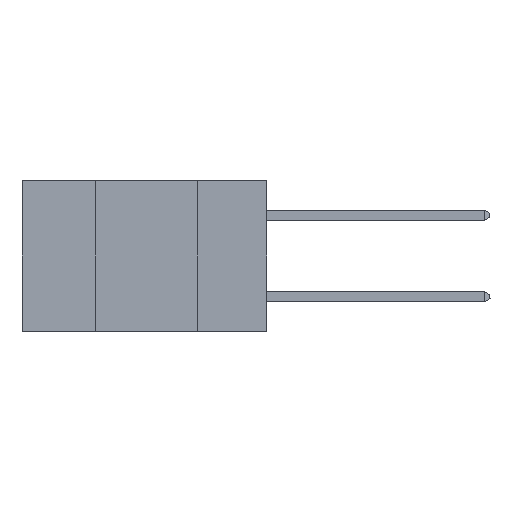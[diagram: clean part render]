
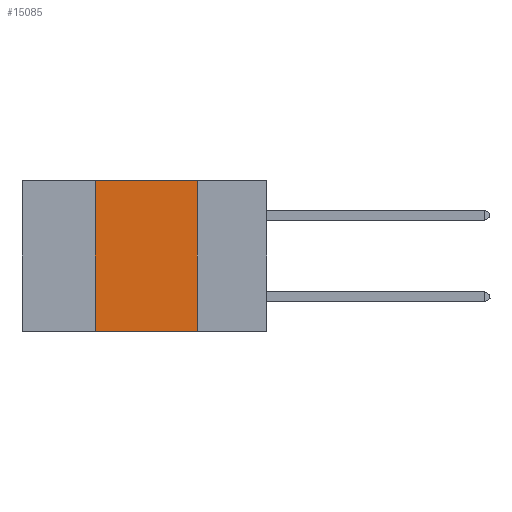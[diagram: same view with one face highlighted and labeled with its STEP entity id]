
A CAD part, left-side view. The second image highlights one B-rep face of the part: STEP entity #15085.
In plain terms, the highlighted planar face has unit normal (-1, 0, 0).
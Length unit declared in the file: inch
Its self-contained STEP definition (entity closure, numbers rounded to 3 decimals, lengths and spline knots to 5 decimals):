
#708 = CARTESIAN_POINT ( 'NONE',  ( 0., 0.6, -0.37 ) ) ;
#858 = CARTESIAN_POINT ( 'NONE',  ( 0., 0.42, 0. ) ) ;
#1692 = VECTOR ( 'NONE', #8683, 39.37008 ) ;
#1806 = ORIENTED_EDGE ( 'NONE', *, *, #21618, .F. ) ;
#2243 = PLANE ( 'NONE',  #3837 ) ;
#3837 = AXIS2_PLACEMENT_3D ( 'NONE', #10097, #6200, #8025 ) ;
#5369 = CARTESIAN_POINT ( 'NONE',  ( 0., 0.42, 0. ) ) ;
#6200 = DIRECTION ( 'NONE',  ( 1., 0., 0. ) ) ;
#6962 = VECTOR ( 'NONE', #6995, 39.37008 ) ;
#6995 = DIRECTION ( 'NONE',  ( 0., -1., 0. ) ) ;
#7097 = DIRECTION ( 'NONE',  ( 0., 0., 1. ) ) ;
#8025 = DIRECTION ( 'NONE',  ( 0., 0., -1. ) ) ;
#8031 = VECTOR ( 'NONE', #7097, 39.37008 ) ;
#8683 = DIRECTION ( 'NONE',  ( 0., -1., 0. ) ) ;
#8914 = CARTESIAN_POINT ( 'NONE',  ( 0., 0.42, -0.37 ) ) ;
#9021 = VERTEX_POINT ( 'NONE', #8914 ) ;
#9606 = EDGE_LOOP ( 'NONE', ( #1806, #12140, #15367, #12699 ) ) ;
#10015 = VERTEX_POINT ( 'NONE', #5369 ) ;
#10097 = CARTESIAN_POINT ( 'NONE',  ( 0., 0.6, 0. ) ) ;
#11702 = DIRECTION ( 'NONE',  ( 0., 0., -1. ) ) ;
#12140 = ORIENTED_EDGE ( 'NONE', *, *, #24425, .F. ) ;
#12699 = ORIENTED_EDGE ( 'NONE', *, *, #23178, .T. ) ;
#13065 = CARTESIAN_POINT ( 'NONE',  ( 0., 0.17, -0.37 ) ) ;
#13338 = VECTOR ( 'NONE', #11702, 39.37008 ) ;
#13755 = CARTESIAN_POINT ( 'NONE',  ( 0., 0.17, 0. ) ) ;
#13918 = LINE ( 'NONE', #858, #8031 ) ;
#14097 = LINE ( 'NONE', #22648, #6962 ) ;
#14491 = EDGE_CURVE ( 'NONE', #9021, #10015, #13918, .T. ) ;
#15085 = ADVANCED_FACE ( 'NONE', ( #20471 ), #2243, .F. ) ;
#15367 = ORIENTED_EDGE ( 'NONE', *, *, #14491, .F. ) ;
#15810 = VERTEX_POINT ( 'NONE', #13065 ) ;
#16928 = VERTEX_POINT ( 'NONE', #20679 ) ;
#18644 = LINE ( 'NONE', #13755, #13338 ) ;
#20390 = LINE ( 'NONE', #708, #1692 ) ;
#20471 = FACE_OUTER_BOUND ( 'NONE', #9606, .T. ) ;
#20679 = CARTESIAN_POINT ( 'NONE',  ( 0., 0.17, 0. ) ) ;
#21618 = EDGE_CURVE ( 'NONE', #16928, #15810, #18644, .T. ) ;
#22648 = CARTESIAN_POINT ( 'NONE',  ( 0., 0.6, 0. ) ) ;
#23178 = EDGE_CURVE ( 'NONE', #9021, #15810, #20390, .T. ) ;
#24425 = EDGE_CURVE ( 'NONE', #10015, #16928, #14097, .T. ) ;
